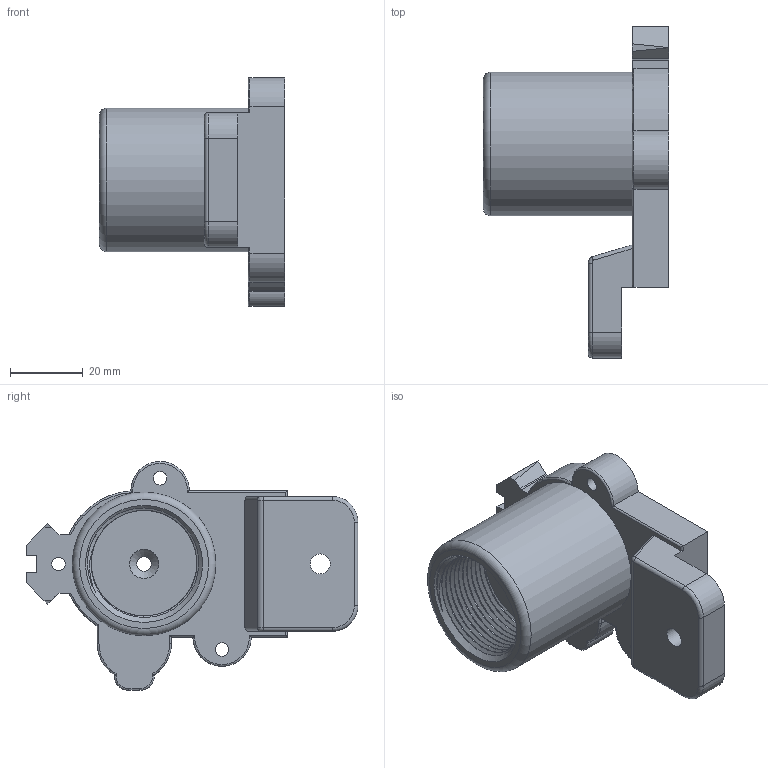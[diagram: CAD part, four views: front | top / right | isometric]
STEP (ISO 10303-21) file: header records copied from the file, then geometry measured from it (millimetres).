
FILE_DESCRIPTION (( 'STEP AP203' ), '1' );
FILE_NAME ('WTF-9_hillbilly_endcap_threaded.STEP', '2020-05-09T08:49:57', ( '' ), ( '' ), 'SwSTEP 2.0', 'SolidWorks 2016', '' );
FILE_SCHEMA (( 'CONFIG_CONTROL_DESIGN' ));
Length unit declared in the file: millimetre
Products named in the file (2): WTF-9_hillbilly_endcap_threaded; WTF HILLBILLY FINAL_8
Assembly tree (1 placements, depth 2):
  WTF-9_hillbilly_endcap_threaded
    WTF HILLBILLY FINAL_8
Bounding box: 50.81 x 91.08 x 62.82 mm (x, y, z)
Volume: 66251.4 mm3; surface area: 21330.6 mm2
Topology: 1 solids, 2 shells, 104 faces, 271 edges, 173 vertices
Faces by surface type: plane 40, cylinder 33, torus 14, bspline 14, cone 3
Full cylindrical faces by diameter (mm): 3.7 x3, 4 x1, 5.5 x1, 22.8 x1, 39.418 x1
Entity records: 12506 total; most frequent: CARTESIAN_POINT 9981, ORIENTED_EDGE 512, DIRECTION 440, EDGE_CURVE 256, VERTEX_POINT 170, AXIS2_PLACEMENT_3D 162, EDGE_LOOP 130, LINE 116
